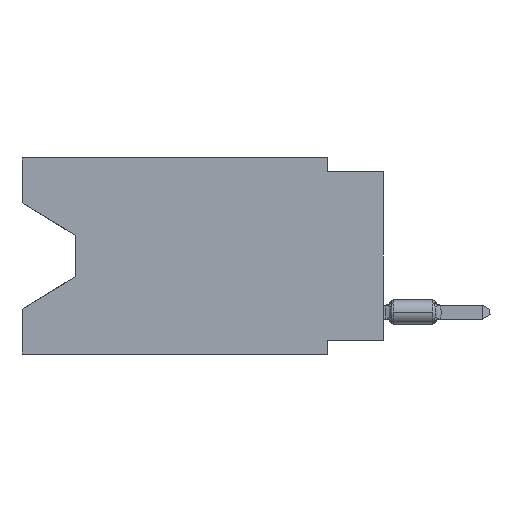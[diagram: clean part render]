
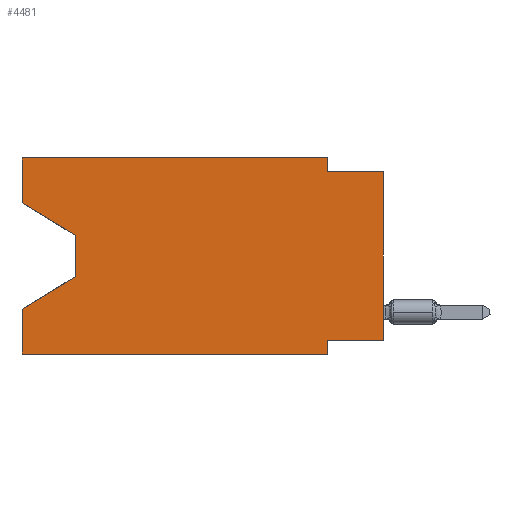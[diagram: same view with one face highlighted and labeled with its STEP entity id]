
A CAD part, left-side view. The second image highlights one B-rep face of the part: STEP entity #4481.
In plain terms, the highlighted planar face has unit normal (-1, 0, 0).
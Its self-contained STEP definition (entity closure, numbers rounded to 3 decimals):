
#149 = DIRECTION ( 'NONE',  ( 1., 0., 0. ) ) ;
#3148 = CARTESIAN_POINT ( 'NONE',  ( 0., 2.54, 0. ) ) ;
#3852 = VERTEX_POINT ( 'NONE', #23904 ) ;
#4481 = ADVANCED_FACE ( 'NONE', ( #5915 ), #80450, .F. ) ;
#5192 = DIRECTION ( 'NONE',  ( 0., 0., -1. ) ) ;
#5915 = FACE_OUTER_BOUND ( 'NONE', #76751, .T. ) ;
#6981 = VECTOR ( 'NONE', #35116, 1000. ) ;
#7415 = EDGE_CURVE ( 'NONE', #3852, #16127, #33144, .T. ) ;
#7545 = LINE ( 'NONE', #57605, #77832 ) ;
#8085 = VERTEX_POINT ( 'NONE', #28639 ) ;
#8597 = CARTESIAN_POINT ( 'NONE',  ( 0., 2.54, -0.635 ) ) ;
#8853 = LINE ( 'NONE', #85633, #6981 ) ;
#9093 = DIRECTION ( 'NONE',  ( 0., -1., 0. ) ) ;
#9963 = CARTESIAN_POINT ( 'NONE',  ( 0., 16.383, 0. ) ) ;
#11054 = ORIENTED_EDGE ( 'NONE', *, *, #87211, .F. ) ;
#12096 = VECTOR ( 'NONE', #85024, 1000. ) ;
#15518 = EDGE_CURVE ( 'NONE', #57752, #77724, #8853, .T. ) ;
#15531 = VECTOR ( 'NONE', #33203, 1000. ) ;
#16127 = VERTEX_POINT ( 'NONE', #52309 ) ;
#16790 = VECTOR ( 'NONE', #60584, 1000. ) ;
#18059 = EDGE_CURVE ( 'NONE', #29103, #16127, #48307, .T. ) ;
#19856 = VECTOR ( 'NONE', #35281, 1000. ) ;
#23904 = CARTESIAN_POINT ( 'NONE',  ( 0., 2.54, -8.255 ) ) ;
#24653 = ORIENTED_EDGE ( 'NONE', *, *, #65936, .F. ) ;
#25363 = LINE ( 'NONE', #68661, #19856 ) ;
#26822 = CARTESIAN_POINT ( 'NONE',  ( 0., 16.383, 0. ) ) ;
#26881 = CARTESIAN_POINT ( 'NONE',  ( 0., 2.54, 0. ) ) ;
#27825 = DIRECTION ( 'NONE',  ( 0., 0., -1. ) ) ;
#28639 = CARTESIAN_POINT ( 'NONE',  ( 0., 13.97, -3.505 ) ) ;
#28811 = EDGE_CURVE ( 'NONE', #72589, #77568, #86023, .T. ) ;
#29103 = VERTEX_POINT ( 'NONE', #54714 ) ;
#31714 = LINE ( 'NONE', #38928, #82547 ) ;
#31720 = VECTOR ( 'NONE', #79519, 1000. ) ;
#33144 = LINE ( 'NONE', #82699, #16790 ) ;
#33203 = DIRECTION ( 'NONE',  ( 0., 0.855, -0.519 ) ) ;
#33628 = CARTESIAN_POINT ( 'NONE',  ( 0., 13.97, -5.385 ) ) ;
#34991 = CARTESIAN_POINT ( 'NONE',  ( 0., 16.383, -2.038 ) ) ;
#35116 = DIRECTION ( 'NONE',  ( 0., 0., 1. ) ) ;
#35281 = DIRECTION ( 'NONE',  ( 0., 1., 0. ) ) ;
#35502 = ORIENTED_EDGE ( 'NONE', *, *, #84968, .F. ) ;
#35773 = EDGE_CURVE ( 'NONE', #86209, #8085, #7545, .T. ) ;
#37170 = LINE ( 'NONE', #66522, #76774 ) ;
#38928 = CARTESIAN_POINT ( 'NONE',  ( 0., 16.383, 0. ) ) ;
#41731 = LINE ( 'NONE', #26822, #70472 ) ;
#43614 = ORIENTED_EDGE ( 'NONE', *, *, #15518, .T. ) ;
#44720 = VERTEX_POINT ( 'NONE', #58764 ) ;
#48307 = LINE ( 'NONE', #86736, #31720 ) ;
#48590 = LINE ( 'NONE', #70682, #15531 ) ;
#49600 = ORIENTED_EDGE ( 'NONE', *, *, #28811, .F. ) ;
#49899 = LINE ( 'NONE', #57116, #12096 ) ;
#52309 = CARTESIAN_POINT ( 'NONE',  ( 0., 2.54, -8.89 ) ) ;
#53032 = VERTEX_POINT ( 'NONE', #33628 ) ;
#54714 = CARTESIAN_POINT ( 'NONE',  ( 0., 16.383, -8.89 ) ) ;
#57116 = CARTESIAN_POINT ( 'NONE',  ( 0., 0., -0.635 ) ) ;
#57605 = CARTESIAN_POINT ( 'NONE',  ( 0., 16.383, -2.038 ) ) ;
#57752 = VERTEX_POINT ( 'NONE', #64170 ) ;
#58339 = CARTESIAN_POINT ( 'NONE',  ( 0., 16.383, 0. ) ) ;
#58764 = CARTESIAN_POINT ( 'NONE',  ( 0., 16.383, -6.852 ) ) ;
#59020 = ORIENTED_EDGE ( 'NONE', *, *, #89370, .T. ) ;
#60461 = ORIENTED_EDGE ( 'NONE', *, *, #68466, .F. ) ;
#60584 = DIRECTION ( 'NONE',  ( 0., 0., -1. ) ) ;
#62837 = ORIENTED_EDGE ( 'NONE', *, *, #18059, .T. ) ;
#64170 = CARTESIAN_POINT ( 'NONE',  ( 0., 0., -8.255 ) ) ;
#65269 = DIRECTION ( 'NONE',  ( 0., 0., 1. ) ) ;
#65936 = EDGE_CURVE ( 'NONE', #91811, #72589, #31714, .T. ) ;
#66276 = EDGE_CURVE ( 'NONE', #8085, #53032, #80194, .T. ) ;
#66522 = CARTESIAN_POINT ( 'NONE',  ( 0., 16.383, 0. ) ) ;
#67283 = ORIENTED_EDGE ( 'NONE', *, *, #7415, .F. ) ;
#68466 = EDGE_CURVE ( 'NONE', #86209, #91811, #37170, .T. ) ;
#68661 = CARTESIAN_POINT ( 'NONE',  ( 0., 0., -8.255 ) ) ;
#69669 = ORIENTED_EDGE ( 'NONE', *, *, #85013, .F. ) ;
#70472 = VECTOR ( 'NONE', #65269, 1000. ) ;
#70682 = CARTESIAN_POINT ( 'NONE',  ( 0., 13.97, -5.385 ) ) ;
#71550 = CARTESIAN_POINT ( 'NONE',  ( 0., 13.97, -3.505 ) ) ;
#72243 = ORIENTED_EDGE ( 'NONE', *, *, #66276, .T. ) ;
#72589 = VERTEX_POINT ( 'NONE', #3148 ) ;
#74180 = DIRECTION ( 'NONE',  ( 0., 0., 1. ) ) ;
#75103 = ORIENTED_EDGE ( 'NONE', *, *, #35773, .T. ) ;
#76393 = AXIS2_PLACEMENT_3D ( 'NONE', #58339, #149, #93463 ) ;
#76751 = EDGE_LOOP ( 'NONE', ( #75103, #72243, #59020, #35502, #62837, #67283, #11054, #43614, #69669, #49600, #24653, #60461 ) ) ;
#76774 = VECTOR ( 'NONE', #74180, 1000. ) ;
#77568 = VERTEX_POINT ( 'NONE', #8597 ) ;
#77724 = VERTEX_POINT ( 'NONE', #83623 ) ;
#77832 = VECTOR ( 'NONE', #94635, 1000. ) ;
#79519 = DIRECTION ( 'NONE',  ( 0., -1., 0. ) ) ;
#80194 = LINE ( 'NONE', #71550, #91732 ) ;
#80450 = PLANE ( 'NONE',  #76393 ) ;
#80622 = VECTOR ( 'NONE', #27825, 1000. ) ;
#82547 = VECTOR ( 'NONE', #9093, 1000. ) ;
#82699 = CARTESIAN_POINT ( 'NONE',  ( 0., 2.54, -8.89 ) ) ;
#83623 = CARTESIAN_POINT ( 'NONE',  ( 0., 0., -0.635 ) ) ;
#84968 = EDGE_CURVE ( 'NONE', #29103, #44720, #41731, .T. ) ;
#85013 = EDGE_CURVE ( 'NONE', #77568, #77724, #49899, .T. ) ;
#85024 = DIRECTION ( 'NONE',  ( 0., -1., 0. ) ) ;
#85633 = CARTESIAN_POINT ( 'NONE',  ( 0., 0., 0. ) ) ;
#86023 = LINE ( 'NONE', #26881, #80622 ) ;
#86209 = VERTEX_POINT ( 'NONE', #34991 ) ;
#86736 = CARTESIAN_POINT ( 'NONE',  ( 0., 16.383, -8.89 ) ) ;
#87211 = EDGE_CURVE ( 'NONE', #57752, #3852, #25363, .T. ) ;
#89370 = EDGE_CURVE ( 'NONE', #53032, #44720, #48590, .T. ) ;
#91732 = VECTOR ( 'NONE', #5192, 1000. ) ;
#91811 = VERTEX_POINT ( 'NONE', #9963 ) ;
#93463 = DIRECTION ( 'NONE',  ( 0., 0., -1. ) ) ;
#94635 = DIRECTION ( 'NONE',  ( 0., -0.855, -0.519 ) ) ;
